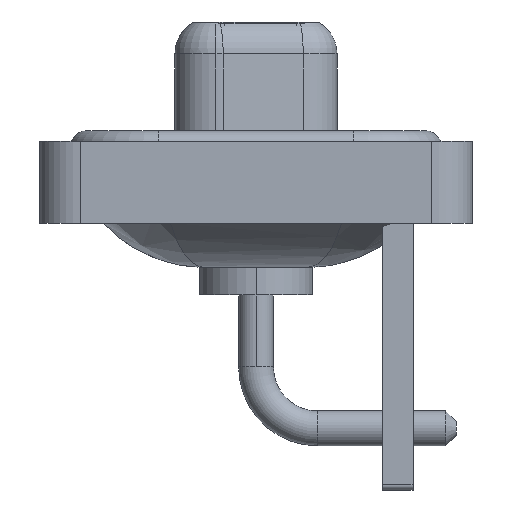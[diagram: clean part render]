
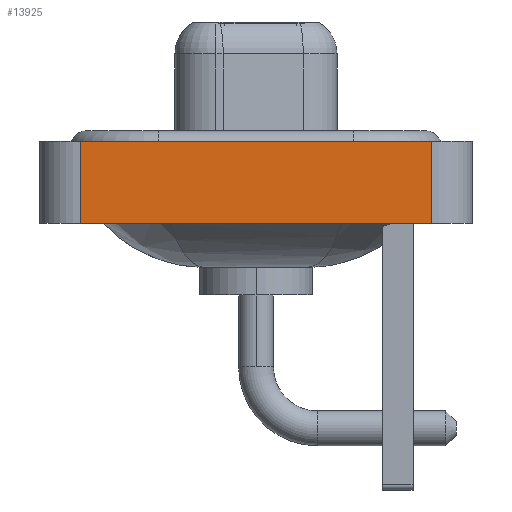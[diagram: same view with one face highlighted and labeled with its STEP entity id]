
A CAD part, left-side view. The second image highlights one B-rep face of the part: STEP entity #13925.
In plain terms, the highlighted planar face has unit normal (-1, 0, 0).
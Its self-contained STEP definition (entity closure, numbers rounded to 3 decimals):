
#460 = EDGE_LOOP ( 'NONE', ( #11423, #2091, #6000, #6317 ) ) ;
#895 = FACE_OUTER_BOUND ( 'NONE', #460, .T. ) ;
#932 = DIRECTION ( 'NONE',  ( 0., 0., 1. ) ) ;
#1664 = CARTESIAN_POINT ( 'NONE',  ( -7.25, 8.55, -3.6 ) ) ;
#1871 = EDGE_CURVE ( 'NONE', #3213, #8500, #11602, .T. ) ;
#2091 = ORIENTED_EDGE ( 'NONE', *, *, #1871, .F. ) ;
#3213 = VERTEX_POINT ( 'NONE', #3988 ) ;
#3988 = CARTESIAN_POINT ( 'NONE',  ( -7.25, 8.55, 0.4 ) ) ;
#4022 = DIRECTION ( 'NONE',  ( 0., -1., 0. ) ) ;
#4661 = LINE ( 'NONE', #8286, #10626 ) ;
#6000 = ORIENTED_EDGE ( 'NONE', *, *, #11913, .F. ) ;
#6050 = PLANE ( 'NONE',  #11708 ) ;
#6317 = ORIENTED_EDGE ( 'NONE', *, *, #14545, .T. ) ;
#8286 = CARTESIAN_POINT ( 'NONE',  ( -7.25, 8.55, -3.6 ) ) ;
#8500 = VERTEX_POINT ( 'NONE', #8639 ) ;
#8639 = CARTESIAN_POINT ( 'NONE',  ( -7.25, -8.55, 0.4 ) ) ;
#8830 = CARTESIAN_POINT ( 'NONE',  ( -7.25, -8.55, -3.6 ) ) ;
#10045 = VECTOR ( 'NONE', #14145, 1000. ) ;
#10594 = CARTESIAN_POINT ( 'NONE',  ( -7.25, -8.55, 0.4 ) ) ;
#10626 = VECTOR ( 'NONE', #14904, 1000. ) ;
#10914 = VECTOR ( 'NONE', #932, 1000. ) ;
#11177 = DIRECTION ( 'NONE',  ( -1., 0., 0. ) ) ;
#11423 = ORIENTED_EDGE ( 'NONE', *, *, #12068, .T. ) ;
#11602 = LINE ( 'NONE', #10594, #10045 ) ;
#11708 = AXIS2_PLACEMENT_3D ( 'NONE', #8830, #11177, #16311 ) ;
#11913 = EDGE_CURVE ( 'NONE', #14169, #3213, #4661, .T. ) ;
#12011 = VERTEX_POINT ( 'NONE', #12298 ) ;
#12068 = EDGE_CURVE ( 'NONE', #12011, #8500, #13912, .T. ) ;
#12298 = CARTESIAN_POINT ( 'NONE',  ( -7.25, -8.55, -3.6 ) ) ;
#12662 = LINE ( 'NONE', #12999, #16573 ) ;
#12999 = CARTESIAN_POINT ( 'NONE',  ( -7.25, -8.55, -3.6 ) ) ;
#13822 = CARTESIAN_POINT ( 'NONE',  ( -7.25, -8.55, -3.6 ) ) ;
#13912 = LINE ( 'NONE', #13822, #10914 ) ;
#13925 = ADVANCED_FACE ( 'NONE', ( #895 ), #6050, .T. ) ;
#14145 = DIRECTION ( 'NONE',  ( 0., -1., 0. ) ) ;
#14169 = VERTEX_POINT ( 'NONE', #1664 ) ;
#14545 = EDGE_CURVE ( 'NONE', #14169, #12011, #12662, .T. ) ;
#14904 = DIRECTION ( 'NONE',  ( 0., 0., 1. ) ) ;
#16311 = DIRECTION ( 'NONE',  ( 0., 0., 1. ) ) ;
#16573 = VECTOR ( 'NONE', #4022, 1000. ) ;
